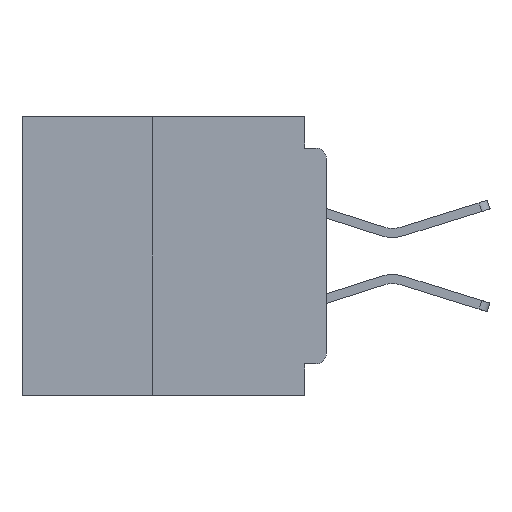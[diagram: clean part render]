
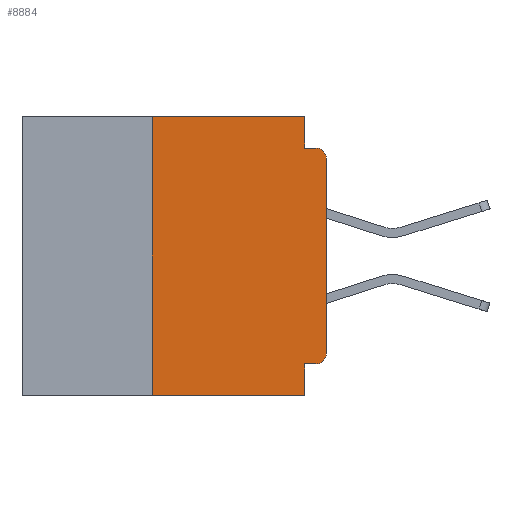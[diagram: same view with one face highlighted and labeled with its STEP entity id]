
A CAD part, left-side view. The second image highlights one B-rep face of the part: STEP entity #8884.
In plain terms, the highlighted planar face has unit normal (-1, 0, 0).
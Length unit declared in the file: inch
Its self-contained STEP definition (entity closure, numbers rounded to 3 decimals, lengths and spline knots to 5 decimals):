
#869 = EDGE_CURVE ( 'NONE', #23967, #24944, #37808, .T. ) ;
#1543 = LINE ( 'NONE', #7683, #42233 ) ;
#1610 = CARTESIAN_POINT ( 'NONE',  ( 0., 0.031, 0. ) ) ;
#1800 = CARTESIAN_POINT ( 'NONE',  ( 0., 0.015, -0.355 ) ) ;
#2363 = LINE ( 'NONE', #45131, #12919 ) ;
#2773 = VERTEX_POINT ( 'NONE', #38808 ) ;
#2823 = VECTOR ( 'NONE', #20099, 39.37008 ) ;
#2869 = ORIENTED_EDGE ( 'NONE', *, *, #47326, .F. ) ;
#3636 = DIRECTION ( 'NONE',  ( 0., 0., -1. ) ) ;
#3676 = DIRECTION ( 'NONE',  ( 0., -1., 0. ) ) ;
#4658 = EDGE_LOOP ( 'NONE', ( #44795, #44804, #37511, #48616, #2869, #13197, #19727, #20224, #9204, #42814 ) ) ;
#4935 = CARTESIAN_POINT ( 'NONE',  ( 0., 0., -0.06 ) ) ;
#5139 = VECTOR ( 'NONE', #29349, 39.37008 ) ;
#5735 = CARTESIAN_POINT ( 'NONE',  ( 0., 0.437, 0. ) ) ;
#7683 = CARTESIAN_POINT ( 'NONE',  ( 0., 0., -0.045 ) ) ;
#8884 = ADVANCED_FACE ( 'NONE', ( #47579 ), #12993, .F. ) ;
#9143 = CARTESIAN_POINT ( 'NONE',  ( 0., 0.031, -0.355 ) ) ;
#9204 = ORIENTED_EDGE ( 'NONE', *, *, #33582, .F. ) ;
#11362 = CARTESIAN_POINT ( 'NONE',  ( 0., 0.031, -0.4 ) ) ;
#12829 = VERTEX_POINT ( 'NONE', #1610 ) ;
#12919 = VECTOR ( 'NONE', #17682, 39.37008 ) ;
#12993 = PLANE ( 'NONE',  #48464 ) ;
#13197 = ORIENTED_EDGE ( 'NONE', *, *, #19840, .F. ) ;
#13700 = CARTESIAN_POINT ( 'NONE',  ( 0., 0.031, -0.4 ) ) ;
#13785 = VERTEX_POINT ( 'NONE', #50388 ) ;
#14022 = VERTEX_POINT ( 'NONE', #9143 ) ;
#16135 = CARTESIAN_POINT ( 'NONE',  ( 0., 0., 0. ) ) ;
#16945 = DIRECTION ( 'NONE',  ( 1., 0., 0. ) ) ;
#17503 = DIRECTION ( 'NONE',  ( 0., 0., -1. ) ) ;
#17682 = DIRECTION ( 'NONE',  ( 0., 0., -1. ) ) ;
#17797 = EDGE_CURVE ( 'NONE', #2773, #24944, #1543, .T. ) ;
#17971 = LINE ( 'NONE', #13700, #37604 ) ;
#18050 = VECTOR ( 'NONE', #23172, 39.37008 ) ;
#19247 = CARTESIAN_POINT ( 'NONE',  ( 0., 0.015, -0.34 ) ) ;
#19727 = ORIENTED_EDGE ( 'NONE', *, *, #32980, .T. ) ;
#19840 = EDGE_CURVE ( 'NONE', #34041, #13785, #28488, .T. ) ;
#20099 = DIRECTION ( 'NONE',  ( 0., 0., 1. ) ) ;
#20224 = ORIENTED_EDGE ( 'NONE', *, *, #38219, .F. ) ;
#22302 = CARTESIAN_POINT ( 'NONE',  ( 0., 0.25, -0.4 ) ) ;
#22475 = EDGE_CURVE ( 'NONE', #12829, #2773, #2363, .T. ) ;
#23170 = DIRECTION ( 'NONE',  ( 0., 0., -1. ) ) ;
#23172 = DIRECTION ( 'NONE',  ( 0., 0., 1. ) ) ;
#23499 = CARTESIAN_POINT ( 'NONE',  ( 0., 0.015, -0.045 ) ) ;
#23557 = DIRECTION ( 'NONE',  ( 0., -1., 0. ) ) ;
#23793 = AXIS2_PLACEMENT_3D ( 'NONE', #39740, #25367, #3636 ) ;
#23967 = VERTEX_POINT ( 'NONE', #4935 ) ;
#24676 = CARTESIAN_POINT ( 'NONE',  ( 0., 0.437, 0. ) ) ;
#24944 = VERTEX_POINT ( 'NONE', #23499 ) ;
#25367 = DIRECTION ( 'NONE',  ( -1., 0., 0. ) ) ;
#27356 = EDGE_CURVE ( 'NONE', #48544, #32060, #33893, .T. ) ;
#27415 = VECTOR ( 'NONE', #47008, 39.37008 ) ;
#28488 = LINE ( 'NONE', #34843, #18050 ) ;
#29277 = EDGE_CURVE ( 'NONE', #32060, #23967, #34277, .T. ) ;
#29349 = DIRECTION ( 'NONE',  ( 0., -1., 0. ) ) ;
#32060 = VERTEX_POINT ( 'NONE', #39593 ) ;
#32904 = VERTEX_POINT ( 'NONE', #11362 ) ;
#32980 = EDGE_CURVE ( 'NONE', #34041, #32904, #47729, .T. ) ;
#33582 = EDGE_CURVE ( 'NONE', #48544, #14022, #39056, .T. ) ;
#33893 = CIRCLE ( 'NONE', #35924, 0.015 ) ;
#34041 = VERTEX_POINT ( 'NONE', #22302 ) ;
#34277 = LINE ( 'NONE', #16135, #2823 ) ;
#34843 = CARTESIAN_POINT ( 'NONE',  ( 0., 0.25, -0.4 ) ) ;
#35392 = CARTESIAN_POINT ( 'NONE',  ( 0., 0.437, -0.4 ) ) ;
#35924 = AXIS2_PLACEMENT_3D ( 'NONE', #19247, #46694, #23170 ) ;
#37274 = VECTOR ( 'NONE', #23557, 39.37008 ) ;
#37511 = ORIENTED_EDGE ( 'NONE', *, *, #17797, .F. ) ;
#37604 = VECTOR ( 'NONE', #17503, 39.37008 ) ;
#37808 = CIRCLE ( 'NONE', #23793, 0.015 ) ;
#38219 = EDGE_CURVE ( 'NONE', #14022, #32904, #17971, .T. ) ;
#38808 = CARTESIAN_POINT ( 'NONE',  ( 0., 0.031, -0.045 ) ) ;
#39056 = LINE ( 'NONE', #43084, #27415 ) ;
#39593 = CARTESIAN_POINT ( 'NONE',  ( 0., 0., -0.34 ) ) ;
#39740 = CARTESIAN_POINT ( 'NONE',  ( 0., 0.015, -0.06 ) ) ;
#42233 = VECTOR ( 'NONE', #3676, 39.37008 ) ;
#42814 = ORIENTED_EDGE ( 'NONE', *, *, #27356, .T. ) ;
#43084 = CARTESIAN_POINT ( 'NONE',  ( 0., 0., -0.355 ) ) ;
#44399 = DIRECTION ( 'NONE',  ( 0., 0., -1. ) ) ;
#44795 = ORIENTED_EDGE ( 'NONE', *, *, #29277, .T. ) ;
#44804 = ORIENTED_EDGE ( 'NONE', *, *, #869, .T. ) ;
#45131 = CARTESIAN_POINT ( 'NONE',  ( 0., 0.031, 0. ) ) ;
#45789 = LINE ( 'NONE', #5735, #5139 ) ;
#46694 = DIRECTION ( 'NONE',  ( -1., 0., 0. ) ) ;
#47008 = DIRECTION ( 'NONE',  ( 0., 1., 0. ) ) ;
#47326 = EDGE_CURVE ( 'NONE', #13785, #12829, #45789, .T. ) ;
#47579 = FACE_OUTER_BOUND ( 'NONE', #4658, .T. ) ;
#47729 = LINE ( 'NONE', #35392, #37274 ) ;
#48464 = AXIS2_PLACEMENT_3D ( 'NONE', #24676, #16945, #44399 ) ;
#48544 = VERTEX_POINT ( 'NONE', #1800 ) ;
#48616 = ORIENTED_EDGE ( 'NONE', *, *, #22475, .F. ) ;
#50388 = CARTESIAN_POINT ( 'NONE',  ( 0., 0.25, 0. ) ) ;
